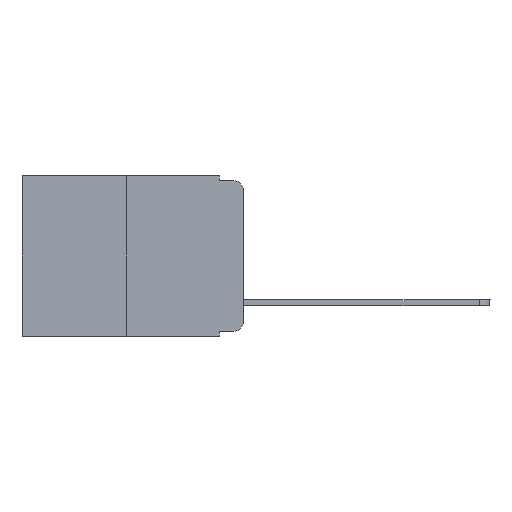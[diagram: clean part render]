
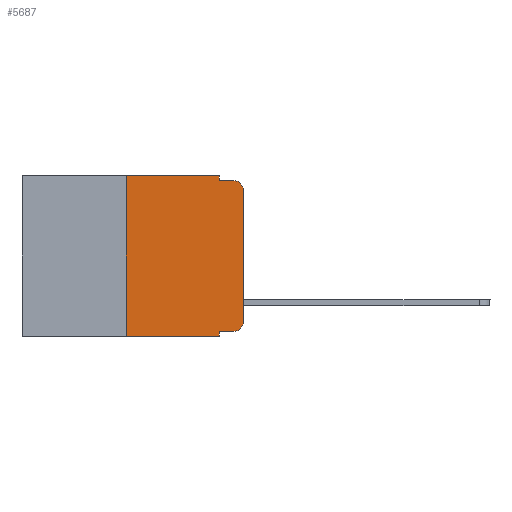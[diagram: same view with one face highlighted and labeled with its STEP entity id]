
A CAD part, left-side view. The second image highlights one B-rep face of the part: STEP entity #5687.
In plain terms, the highlighted planar face has unit normal (-1, 0, 0).
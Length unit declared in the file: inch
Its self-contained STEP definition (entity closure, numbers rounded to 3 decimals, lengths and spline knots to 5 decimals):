
#52 = ORIENTED_EDGE ( 'NONE', *, *, #12562, .T. ) ;
#148 = DIRECTION ( 'NONE',  ( 0., 0., -1. ) ) ;
#473 = VERTEX_POINT ( 'NONE', #5712 ) ;
#729 = VERTEX_POINT ( 'NONE', #3544 ) ;
#884 = CARTESIAN_POINT ( 'NONE',  ( 0., 0.25, -0.343 ) ) ;
#1126 = AXIS2_PLACEMENT_3D ( 'NONE', #11506, #19176, #17592 ) ;
#1298 = EDGE_CURVE ( 'NONE', #9693, #18377, #17655, .T. ) ;
#1439 = AXIS2_PLACEMENT_3D ( 'NONE', #8377, #2275, #10021 ) ;
#1784 = EDGE_CURVE ( 'NONE', #1972, #17972, #16685, .T. ) ;
#1972 = VERTEX_POINT ( 'NONE', #13286 ) ;
#2006 = CARTESIAN_POINT ( 'NONE',  ( 0., 0.051, 0. ) ) ;
#2275 = DIRECTION ( 'NONE',  ( -1., 0., 0. ) ) ;
#2675 = VECTOR ( 'NONE', #3037, 39.37008 ) ;
#2995 = VECTOR ( 'NONE', #5610, 39.37008 ) ;
#3037 = DIRECTION ( 'NONE',  ( 0., 0., 1. ) ) ;
#3361 = EDGE_CURVE ( 'NONE', #9913, #729, #17858, .T. ) ;
#3395 = CARTESIAN_POINT ( 'NONE',  ( 0., 0.051, -0.333 ) ) ;
#3544 = CARTESIAN_POINT ( 'NONE',  ( 0., 0.25, 0. ) ) ;
#3980 = LINE ( 'NONE', #17856, #13866 ) ;
#4764 = CARTESIAN_POINT ( 'NONE',  ( 0., 0.473, -0.343 ) ) ;
#5065 = CARTESIAN_POINT ( 'NONE',  ( 0., 0.051, -0.01 ) ) ;
#5185 = ORIENTED_EDGE ( 'NONE', *, *, #1298, .F. ) ;
#5205 = VECTOR ( 'NONE', #9783, 39.37008 ) ;
#5328 = VECTOR ( 'NONE', #15807, 39.37008 ) ;
#5344 = DIRECTION ( 'NONE',  ( 0., 0., -1. ) ) ;
#5545 = CARTESIAN_POINT ( 'NONE',  ( 0., 0.051, 0. ) ) ;
#5610 = DIRECTION ( 'NONE',  ( 0., 0., -1. ) ) ;
#5687 = ADVANCED_FACE ( 'NONE', ( #6918 ), #11575, .F. ) ;
#5712 = CARTESIAN_POINT ( 'NONE',  ( 0., 0., -0.03 ) ) ;
#5787 = AXIS2_PLACEMENT_3D ( 'NONE', #12153, #6183, #148 ) ;
#6183 = DIRECTION ( 'NONE',  ( -1., 0., 0. ) ) ;
#6564 = LINE ( 'NONE', #11738, #9625 ) ;
#6918 = FACE_OUTER_BOUND ( 'NONE', #11734, .T. ) ;
#7477 = EDGE_CURVE ( 'NONE', #12079, #16688, #19320, .T. ) ;
#7530 = VECTOR ( 'NONE', #5344, 39.37008 ) ;
#7734 = ORIENTED_EDGE ( 'NONE', *, *, #10581, .F. ) ;
#8041 = ORIENTED_EDGE ( 'NONE', *, *, #3361, .F. ) ;
#8377 = CARTESIAN_POINT ( 'NONE',  ( 0., 0.02, -0.313 ) ) ;
#8584 = ORIENTED_EDGE ( 'NONE', *, *, #19193, .T. ) ;
#8848 = VECTOR ( 'NONE', #9277, 39.37008 ) ;
#9070 = EDGE_CURVE ( 'NONE', #16688, #17999, #16310, .T. ) ;
#9277 = DIRECTION ( 'NONE',  ( 0., -1., 0. ) ) ;
#9625 = VECTOR ( 'NONE', #16246, 39.37008 ) ;
#9693 = VERTEX_POINT ( 'NONE', #3395 ) ;
#9783 = DIRECTION ( 'NONE',  ( 0., -1., 0. ) ) ;
#9913 = VERTEX_POINT ( 'NONE', #884 ) ;
#10021 = DIRECTION ( 'NONE',  ( 0., 0., -1. ) ) ;
#10073 = EDGE_CURVE ( 'NONE', #9693, #1972, #3980, .T. ) ;
#10581 = EDGE_CURVE ( 'NONE', #729, #12079, #6564, .T. ) ;
#11506 = CARTESIAN_POINT ( 'NONE',  ( 0., 0.473, 0. ) ) ;
#11575 = PLANE ( 'NONE',  #1126 ) ;
#11734 = EDGE_LOOP ( 'NONE', ( #8584, #12422, #15671, #17269, #7734, #8041, #52, #5185, #14211, #13195 ) ) ;
#11738 = CARTESIAN_POINT ( 'NONE',  ( 0., 0.473, 0. ) ) ;
#12079 = VERTEX_POINT ( 'NONE', #2006 ) ;
#12153 = CARTESIAN_POINT ( 'NONE',  ( 0., 0.02, -0.03 ) ) ;
#12422 = ORIENTED_EDGE ( 'NONE', *, *, #14402, .T. ) ;
#12562 = EDGE_CURVE ( 'NONE', #9913, #18377, #17812, .T. ) ;
#13080 = CARTESIAN_POINT ( 'NONE',  ( 0., 0.051, -0.343 ) ) ;
#13195 = ORIENTED_EDGE ( 'NONE', *, *, #1784, .T. ) ;
#13286 = CARTESIAN_POINT ( 'NONE',  ( 0., 0.02, -0.333 ) ) ;
#13473 = CIRCLE ( 'NONE', #5787, 0.02 ) ;
#13721 = CARTESIAN_POINT ( 'NONE',  ( 0., 0., -0.313 ) ) ;
#13866 = VECTOR ( 'NONE', #19424, 39.37008 ) ;
#14195 = CARTESIAN_POINT ( 'NONE',  ( 0., 0.25, 0. ) ) ;
#14211 = ORIENTED_EDGE ( 'NONE', *, *, #10073, .T. ) ;
#14402 = EDGE_CURVE ( 'NONE', #473, #17999, #13473, .T. ) ;
#15671 = ORIENTED_EDGE ( 'NONE', *, *, #9070, .F. ) ;
#15807 = DIRECTION ( 'NONE',  ( 0., 0., 1. ) ) ;
#16246 = DIRECTION ( 'NONE',  ( 0., -1., 0. ) ) ;
#16310 = LINE ( 'NONE', #5065, #5205 ) ;
#16685 = CIRCLE ( 'NONE', #1439, 0.02 ) ;
#16688 = VERTEX_POINT ( 'NONE', #19433 ) ;
#16778 = CARTESIAN_POINT ( 'NONE',  ( 0., 0., 0. ) ) ;
#17269 = ORIENTED_EDGE ( 'NONE', *, *, #7477, .F. ) ;
#17592 = DIRECTION ( 'NONE',  ( 0., 0., -1. ) ) ;
#17655 = LINE ( 'NONE', #5545, #2995 ) ;
#17812 = LINE ( 'NONE', #4764, #8848 ) ;
#17856 = CARTESIAN_POINT ( 'NONE',  ( 0., 0.051, -0.333 ) ) ;
#17858 = LINE ( 'NONE', #14195, #5328 ) ;
#17972 = VERTEX_POINT ( 'NONE', #13721 ) ;
#17999 = VERTEX_POINT ( 'NONE', #18793 ) ;
#18278 = LINE ( 'NONE', #16778, #2675 ) ;
#18377 = VERTEX_POINT ( 'NONE', #13080 ) ;
#18793 = CARTESIAN_POINT ( 'NONE',  ( 0., 0.02, -0.01 ) ) ;
#19149 = CARTESIAN_POINT ( 'NONE',  ( 0., 0.051, 0. ) ) ;
#19176 = DIRECTION ( 'NONE',  ( 1., 0., 0. ) ) ;
#19193 = EDGE_CURVE ( 'NONE', #17972, #473, #18278, .T. ) ;
#19320 = LINE ( 'NONE', #19149, #7530 ) ;
#19424 = DIRECTION ( 'NONE',  ( 0., -1., 0. ) ) ;
#19433 = CARTESIAN_POINT ( 'NONE',  ( 0., 0.051, -0.01 ) ) ;
